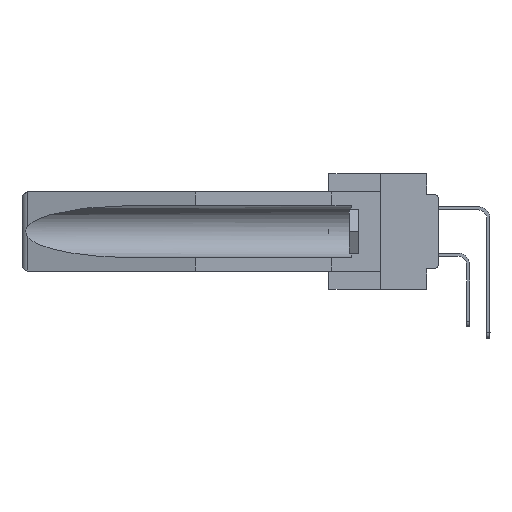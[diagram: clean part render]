
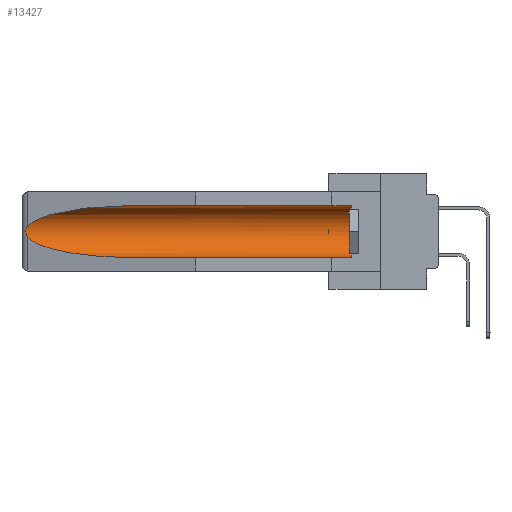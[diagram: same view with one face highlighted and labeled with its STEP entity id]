
A CAD part, left-side view. The second image highlights one B-rep face of the part: STEP entity #13427.
In plain terms, the highlighted cylindrical face has radius 2.857 mm (diameter 5.715 mm), a partial arc.
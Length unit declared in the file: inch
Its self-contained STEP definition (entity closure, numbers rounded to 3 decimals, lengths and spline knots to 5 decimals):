
#631 = VERTEX_POINT ( 'NONE', #20172 ) ;
#1444 = DIRECTION ( 'NONE',  ( 0., 1., 0. ) ) ;
#1733 = CARTESIAN_POINT ( 'NONE',  ( 0.26597, 1.52961, -0.15275 ) ) ;
#2335 = AXIS2_PLACEMENT_3D ( 'NONE', #20715, #34303, #11120 ) ;
#2541 = CARTESIAN_POINT ( 'NONE',  ( 0.26537, 1.52718, -0.14972 ) ) ;
#4278 = CARTESIAN_POINT ( 'NONE',  ( 0.26537, 1.52718, -0.14972 ) ) ;
#4691 = CARTESIAN_POINT ( 'NONE',  ( 0.26655, 1.53094, -0.18657 ) ) ;
#5144 = CYLINDRICAL_SURFACE ( 'NONE', #2335, 0.1125 ) ;
#6048 =( BOUNDED_CURVE ( )  B_SPLINE_CURVE ( 3, ( #31057, #28073, #27656, #2541 ),
 .UNSPECIFIED., .F., .T. ) 
 B_SPLINE_CURVE_WITH_KNOTS ( ( 4, 4 ),
 ( 4.71239, 6.08839 ),
 .UNSPECIFIED. ) 
 CURVE ( )  GEOMETRIC_REPRESENTATION_ITEM ( )  RATIONAL_B_SPLINE_CURVE ( ( 1., 0.848, 0.848, 1. ) ) 
 REPRESENTATION_ITEM ( '' )  );
#7762 = LINE ( 'NONE', #20762, #28690 ) ;
#8277 = CARTESIAN_POINT ( 'NONE',  ( 0.26537, 1.52718, -0.19328 ) ) ;
#11120 = DIRECTION ( 'NONE',  ( 0., 0., 1. ) ) ;
#11351 = ORIENTED_EDGE ( 'NONE', *, *, #14205, .T. ) ;
#11898 = CARTESIAN_POINT ( 'NONE',  ( 0.155, 1.07973, -0.284 ) ) ;
#13427 = ADVANCED_FACE ( 'NONE', ( #33878 ), #5144, .F. ) ;
#14205 = EDGE_CURVE ( 'NONE', #39521, #41731, #23564, .T. ) ;
#14426 = ORIENTED_EDGE ( 'NONE', *, *, #25377, .T. ) ;
#14695 = CARTESIAN_POINT ( 'NONE',  ( 0.26597, 1.5296, -0.19026 ) ) ;
#15414 = ORIENTED_EDGE ( 'NONE', *, *, #34263, .T. ) ;
#17274 = CARTESIAN_POINT ( 'NONE',  ( 0.2673, 1.53269, -0.17917 ) ) ;
#17489 = CARTESIAN_POINT ( 'NONE',  ( 0.2673, 1.5327, -0.16383 ) ) ;
#17669 = CARTESIAN_POINT ( 'NONE',  ( 0.155, 1.07973, -0.284 ) ) ;
#19958 = EDGE_LOOP ( 'NONE', ( #27715, #34749, #14426, #20394, #15414, #11351 ) ) ;
#20172 = CARTESIAN_POINT ( 'NONE',  ( 0.26537, 1.52718, -0.14972 ) ) ;
#20394 = ORIENTED_EDGE ( 'NONE', *, *, #35887, .F. ) ;
#20715 = CARTESIAN_POINT ( 'NONE',  ( 0.155, -0.30754, -0.1715 ) ) ;
#20762 = CARTESIAN_POINT ( 'NONE',  ( 0.155, -0.30754, -0.284 ) ) ;
#20899 = CARTESIAN_POINT ( 'NONE',  ( 0.2675, 1.53308, -0.16763 ) ) ;
#20963 = DIRECTION ( 'NONE',  ( 0., 1., 0. ) ) ;
#21247 = VERTEX_POINT ( 'NONE', #17669 ) ;
#23468 = EDGE_CURVE ( 'NONE', #631, #36812, #25299, .T. ) ;
#23564 = LINE ( 'NONE', #40172, #41026 ) ;
#24862 = CARTESIAN_POINT ( 'NONE',  ( 0.21114, 1.30732, -0.284 ) ) ;
#25278 = CARTESIAN_POINT ( 'NONE',  ( 0.25451, 1.48313, -0.24835 ) ) ;
#25299 = B_SPLINE_CURVE_WITH_KNOTS ( 'NONE', 3,
 ( #4278, #1733, #33428, #17489, #20899, #33652, #17274, #4691, #14695, #40258 ),
 .UNSPECIFIED., .F., .F.,
 ( 4, 2, 2, 2, 4 ),
 ( 0., 0.00029, 0.00058, 0.00087, 0.00117 ),
 .UNSPECIFIED. ) ;
#25377 = EDGE_CURVE ( 'NONE', #36812, #21247, #30768, .T. ) ;
#27655 = CARTESIAN_POINT ( 'NONE',  ( 0.155, 0.126, -0.1715 ) ) ;
#27656 = CARTESIAN_POINT ( 'NONE',  ( 0.25451, 1.48313, -0.09465 ) ) ;
#27715 = ORIENTED_EDGE ( 'NONE', *, *, #39445, .T. ) ;
#28073 = CARTESIAN_POINT ( 'NONE',  ( 0.21114, 1.30732, -0.059 ) ) ;
#28690 = VECTOR ( 'NONE', #20963, 39.37008 ) ;
#30637 = CIRCLE ( 'NONE', #37447, 0.1125 ) ;
#30768 =( BOUNDED_CURVE ( )  B_SPLINE_CURVE ( 3, ( #8277, #25278, #24862, #11898 ),
 .UNSPECIFIED., .F., .T. ) 
 B_SPLINE_CURVE_WITH_KNOTS ( ( 4, 4 ),
 ( 0.1948, 1.5708 ),
 .UNSPECIFIED. ) 
 CURVE ( )  GEOMETRIC_REPRESENTATION_ITEM ( )  RATIONAL_B_SPLINE_CURVE ( ( 1., 0.848, 0.848, 1. ) ) 
 REPRESENTATION_ITEM ( '' )  );
#31057 = CARTESIAN_POINT ( 'NONE',  ( 0.155, 1.07973, -0.059 ) ) ;
#31062 = VERTEX_POINT ( 'NONE', #34798 ) ;
#33428 = CARTESIAN_POINT ( 'NONE',  ( 0.26654, 1.53092, -0.15636 ) ) ;
#33652 = CARTESIAN_POINT ( 'NONE',  ( 0.2675, 1.53308, -0.17534 ) ) ;
#33832 = DIRECTION ( 'NONE',  ( 0., 0., 1. ) ) ;
#33878 = FACE_OUTER_BOUND ( 'NONE', #19958, .T. ) ;
#34263 = EDGE_CURVE ( 'NONE', #31062, #39521, #30637, .T. ) ;
#34303 = DIRECTION ( 'NONE',  ( 0., 1., 0. ) ) ;
#34749 = ORIENTED_EDGE ( 'NONE', *, *, #23468, .T. ) ;
#34798 = CARTESIAN_POINT ( 'NONE',  ( 0.155, 0.126, -0.284 ) ) ;
#35236 = CARTESIAN_POINT ( 'NONE',  ( 0.26537, 1.52718, -0.19328 ) ) ;
#35887 = EDGE_CURVE ( 'NONE', #31062, #21247, #7762, .T. ) ;
#36428 = CARTESIAN_POINT ( 'NONE',  ( 0.155, 1.07973, -0.059 ) ) ;
#36812 = VERTEX_POINT ( 'NONE', #35236 ) ;
#37447 = AXIS2_PLACEMENT_3D ( 'NONE', #27655, #40868, #33832 ) ;
#39445 = EDGE_CURVE ( 'NONE', #41731, #631, #6048, .T. ) ;
#39521 = VERTEX_POINT ( 'NONE', #40869 ) ;
#40172 = CARTESIAN_POINT ( 'NONE',  ( 0.155, -0.30754, -0.059 ) ) ;
#40258 = CARTESIAN_POINT ( 'NONE',  ( 0.26537, 1.52718, -0.19328 ) ) ;
#40868 = DIRECTION ( 'NONE',  ( 0., -1., 0. ) ) ;
#40869 = CARTESIAN_POINT ( 'NONE',  ( 0.155, 0.126, -0.059 ) ) ;
#41026 = VECTOR ( 'NONE', #1444, 39.37008 ) ;
#41731 = VERTEX_POINT ( 'NONE', #36428 ) ;
